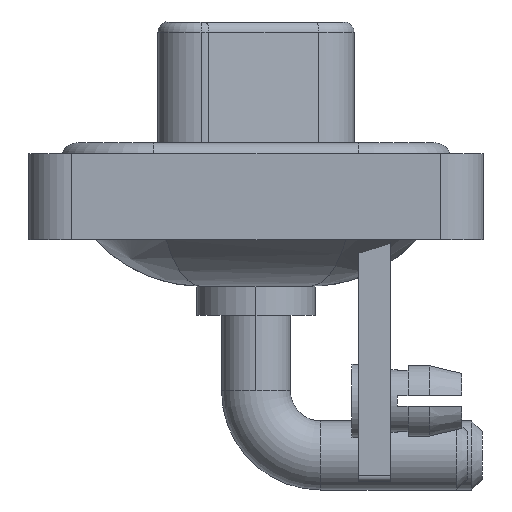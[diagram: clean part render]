
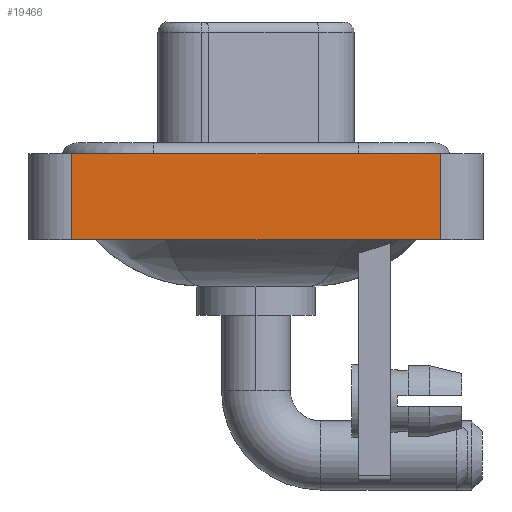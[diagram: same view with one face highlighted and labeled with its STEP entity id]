
A CAD part, left-side view. The second image highlights one B-rep face of the part: STEP entity #19466.
In plain terms, the highlighted planar face has unit normal (-1, 0, 0).
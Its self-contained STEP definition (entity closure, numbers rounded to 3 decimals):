
#139 = EDGE_CURVE ( 'NONE', #1588, #7466, #2184, .T. ) ;
#528 = DIRECTION ( 'NONE',  ( 0., 0., 1. ) ) ;
#955 = EDGE_CURVE ( 'NONE', #1455, #2147, #9543, .T. ) ;
#1198 = EDGE_LOOP ( 'NONE', ( #4929, #16534, #18560, #19764 ) ) ;
#1291 = CARTESIAN_POINT ( 'NONE',  ( -7.3, -8.55, -3.6 ) ) ;
#1300 = CARTESIAN_POINT ( 'NONE',  ( -7.3, 8.55, -3.6 ) ) ;
#1455 = VERTEX_POINT ( 'NONE', #1300 ) ;
#1515 = AXIS2_PLACEMENT_3D ( 'NONE', #1291, #9618, #18085 ) ;
#1588 = VERTEX_POINT ( 'NONE', #5006 ) ;
#1777 = LINE ( 'NONE', #6818, #10975 ) ;
#1838 = CARTESIAN_POINT ( 'NONE',  ( -7.3, -8.55, -3.6 ) ) ;
#2147 = VERTEX_POINT ( 'NONE', #15946 ) ;
#2184 = LINE ( 'NONE', #12134, #21598 ) ;
#3022 = VECTOR ( 'NONE', #5938, 1000. ) ;
#4355 = CARTESIAN_POINT ( 'NONE',  ( -7.3, -8.55, 0.4 ) ) ;
#4929 = ORIENTED_EDGE ( 'NONE', *, *, #139, .T. ) ;
#5006 = CARTESIAN_POINT ( 'NONE',  ( -7.3, -8.55, -3.6 ) ) ;
#5657 = VECTOR ( 'NONE', #15222, 1000. ) ;
#5938 = DIRECTION ( 'NONE',  ( 0., 0., 1. ) ) ;
#6775 = LINE ( 'NONE', #1838, #5657 ) ;
#6818 = CARTESIAN_POINT ( 'NONE',  ( -7.3, -8.55, 0.4 ) ) ;
#7466 = VERTEX_POINT ( 'NONE', #4355 ) ;
#9543 = LINE ( 'NONE', #16132, #3022 ) ;
#9618 = DIRECTION ( 'NONE',  ( -1., 0., 0. ) ) ;
#10975 = VECTOR ( 'NONE', #16822, 1000. ) ;
#11251 = FACE_OUTER_BOUND ( 'NONE', #1198, .T. ) ;
#12134 = CARTESIAN_POINT ( 'NONE',  ( -7.3, -8.55, -3.6 ) ) ;
#12346 = EDGE_CURVE ( 'NONE', #2147, #7466, #1777, .T. ) ;
#15222 = DIRECTION ( 'NONE',  ( 0., -1., 0. ) ) ;
#15946 = CARTESIAN_POINT ( 'NONE',  ( -7.3, 8.55, 0.4 ) ) ;
#16132 = CARTESIAN_POINT ( 'NONE',  ( -7.3, 8.55, -3.6 ) ) ;
#16534 = ORIENTED_EDGE ( 'NONE', *, *, #12346, .F. ) ;
#16664 = EDGE_CURVE ( 'NONE', #1455, #1588, #6775, .T. ) ;
#16822 = DIRECTION ( 'NONE',  ( 0., -1., 0. ) ) ;
#17872 = PLANE ( 'NONE',  #1515 ) ;
#18085 = DIRECTION ( 'NONE',  ( 0., 0., 1. ) ) ;
#18560 = ORIENTED_EDGE ( 'NONE', *, *, #955, .F. ) ;
#19466 = ADVANCED_FACE ( 'NONE', ( #11251 ), #17872, .T. ) ;
#19764 = ORIENTED_EDGE ( 'NONE', *, *, #16664, .T. ) ;
#21598 = VECTOR ( 'NONE', #528, 1000. ) ;
